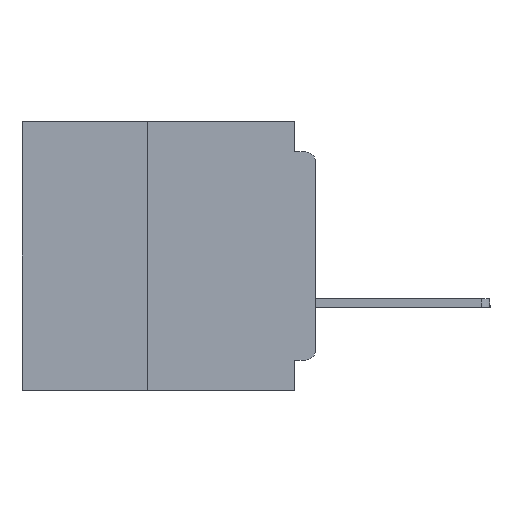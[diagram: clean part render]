
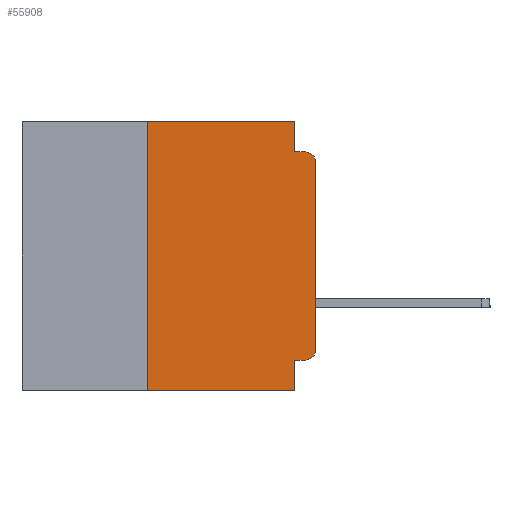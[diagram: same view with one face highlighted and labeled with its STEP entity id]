
A CAD part, left-side view. The second image highlights one B-rep face of the part: STEP entity #55908.
In plain terms, the highlighted planar face has unit normal (-1, 0, 0).
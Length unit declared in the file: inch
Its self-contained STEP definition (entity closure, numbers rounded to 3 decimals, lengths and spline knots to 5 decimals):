
#20 = VERTEX_POINT ( 'NONE', #24522 ) ;
#224 = CARTESIAN_POINT ( 'NONE',  ( 0., 0.015, -0.06 ) ) ;
#726 = LINE ( 'NONE', #30861, #12191 ) ;
#818 = CARTESIAN_POINT ( 'NONE',  ( 0., 0.437, 0. ) ) ;
#1888 = DIRECTION ( 'NONE',  ( 0., -1., 0. ) ) ;
#3076 = ORIENTED_EDGE ( 'NONE', *, *, #14187, .F. ) ;
#3873 = VERTEX_POINT ( 'NONE', #3890 ) ;
#3890 = CARTESIAN_POINT ( 'NONE',  ( 0., 0., -0.06 ) ) ;
#4310 = DIRECTION ( 'NONE',  ( -1., 0., 0. ) ) ;
#5172 = DIRECTION ( 'NONE',  ( 0., 0., -1. ) ) ;
#5753 = DIRECTION ( 'NONE',  ( 0., 0., -1. ) ) ;
#6832 = ORIENTED_EDGE ( 'NONE', *, *, #9218, .F. ) ;
#8948 = VERTEX_POINT ( 'NONE', #24760 ) ;
#9218 = EDGE_CURVE ( 'NONE', #56957, #15188, #60233, .T. ) ;
#9651 = VECTOR ( 'NONE', #26650, 39.37008 ) ;
#9914 = VERTEX_POINT ( 'NONE', #55533 ) ;
#10625 = ORIENTED_EDGE ( 'NONE', *, *, #50321, .F. ) ;
#11396 = ORIENTED_EDGE ( 'NONE', *, *, #52573, .F. ) ;
#12191 = VECTOR ( 'NONE', #16539, 39.37008 ) ;
#12241 = EDGE_CURVE ( 'NONE', #8948, #20674, #726, .T. ) ;
#12312 = CARTESIAN_POINT ( 'NONE',  ( 0., 0., -0.355 ) ) ;
#12936 = EDGE_LOOP ( 'NONE', ( #21149, #47153, #47600, #10625, #11396, #6832, #40379, #48515, #3076, #17005 ) ) ;
#14187 = EDGE_CURVE ( 'NONE', #20, #8948, #46287, .T. ) ;
#14747 = CARTESIAN_POINT ( 'NONE',  ( 0., 0.031, -0.4 ) ) ;
#15188 = VERTEX_POINT ( 'NONE', #15337 ) ;
#15337 = CARTESIAN_POINT ( 'NONE',  ( 0., 0.25, 0. ) ) ;
#16345 = CARTESIAN_POINT ( 'NONE',  ( 0., 0., -0.045 ) ) ;
#16539 = DIRECTION ( 'NONE',  ( 0., 0., -1. ) ) ;
#17005 = ORIENTED_EDGE ( 'NONE', *, *, #46021, .T. ) ;
#20462 = LINE ( 'NONE', #60991, #55417 ) ;
#20674 = VERTEX_POINT ( 'NONE', #14747 ) ;
#21149 = ORIENTED_EDGE ( 'NONE', *, *, #46573, .T. ) ;
#21514 = EDGE_CURVE ( 'NONE', #9914, #60119, #39062, .T. ) ;
#22411 = VECTOR ( 'NONE', #31202, 39.37008 ) ;
#24050 = CARTESIAN_POINT ( 'NONE',  ( 0., 0.031, 0. ) ) ;
#24522 = CARTESIAN_POINT ( 'NONE',  ( 0., 0.015, -0.355 ) ) ;
#24693 = AXIS2_PLACEMENT_3D ( 'NONE', #33201, #4310, #37907 ) ;
#24760 = CARTESIAN_POINT ( 'NONE',  ( 0., 0.031, -0.355 ) ) ;
#26650 = DIRECTION ( 'NONE',  ( 0., 1., 0. ) ) ;
#28067 = CIRCLE ( 'NONE', #24693, 0.015 ) ;
#30284 = CIRCLE ( 'NONE', #51730, 0.015 ) ;
#30861 = CARTESIAN_POINT ( 'NONE',  ( 0., 0.031, -0.4 ) ) ;
#31202 = DIRECTION ( 'NONE',  ( 0., 0., 1. ) ) ;
#32042 = VERTEX_POINT ( 'NONE', #36938 ) ;
#32251 = LINE ( 'NONE', #24050, #55947 ) ;
#32519 = FACE_OUTER_BOUND ( 'NONE', #12936, .T. ) ;
#33201 = CARTESIAN_POINT ( 'NONE',  ( 0., 0.015, -0.34 ) ) ;
#33380 = DIRECTION ( 'NONE',  ( 0., -1., 0. ) ) ;
#33451 = VERTEX_POINT ( 'NONE', #48397 ) ;
#34052 = DIRECTION ( 'NONE',  ( -1., 0., 0. ) ) ;
#34593 = DIRECTION ( 'NONE',  ( 1., 0., 0. ) ) ;
#36938 = CARTESIAN_POINT ( 'NONE',  ( 0., 0., -0.34 ) ) ;
#37600 = VECTOR ( 'NONE', #1888, 39.37008 ) ;
#37907 = DIRECTION ( 'NONE',  ( 0., 0., -1. ) ) ;
#38550 = LINE ( 'NONE', #61639, #52707 ) ;
#39062 = LINE ( 'NONE', #16345, #37600 ) ;
#40379 = ORIENTED_EDGE ( 'NONE', *, *, #50303, .T. ) ;
#42589 = CARTESIAN_POINT ( 'NONE',  ( 0., 0.25, -0.4 ) ) ;
#43117 = DIRECTION ( 'NONE',  ( 0., 0., -1. ) ) ;
#46021 = EDGE_CURVE ( 'NONE', #20, #32042, #28067, .T. ) ;
#46287 = LINE ( 'NONE', #12312, #9651 ) ;
#46304 = LINE ( 'NONE', #47697, #57376 ) ;
#46573 = EDGE_CURVE ( 'NONE', #32042, #3873, #20462, .T. ) ;
#47153 = ORIENTED_EDGE ( 'NONE', *, *, #59914, .T. ) ;
#47600 = ORIENTED_EDGE ( 'NONE', *, *, #21514, .F. ) ;
#47697 = CARTESIAN_POINT ( 'NONE',  ( 0., 0.437, -0.4 ) ) ;
#48397 = CARTESIAN_POINT ( 'NONE',  ( 0., 0.031, 0. ) ) ;
#48515 = ORIENTED_EDGE ( 'NONE', *, *, #12241, .F. ) ;
#50303 = EDGE_CURVE ( 'NONE', #56957, #20674, #46304, .T. ) ;
#50321 = EDGE_CURVE ( 'NONE', #33451, #9914, #32251, .T. ) ;
#51730 = AXIS2_PLACEMENT_3D ( 'NONE', #224, #34052, #5172 ) ;
#52505 = DIRECTION ( 'NONE',  ( 0., -1., 0. ) ) ;
#52573 = EDGE_CURVE ( 'NONE', #15188, #33451, #38550, .T. ) ;
#52707 = VECTOR ( 'NONE', #33380, 39.37008 ) ;
#55305 = AXIS2_PLACEMENT_3D ( 'NONE', #818, #34593, #5753 ) ;
#55417 = VECTOR ( 'NONE', #56299, 39.37008 ) ;
#55533 = CARTESIAN_POINT ( 'NONE',  ( 0., 0.031, -0.045 ) ) ;
#55908 = ADVANCED_FACE ( 'NONE', ( #32519 ), #58139, .F. ) ;
#55947 = VECTOR ( 'NONE', #43117, 39.37008 ) ;
#56299 = DIRECTION ( 'NONE',  ( 0., 0., 1. ) ) ;
#56957 = VERTEX_POINT ( 'NONE', #42589 ) ;
#57376 = VECTOR ( 'NONE', #52505, 39.37008 ) ;
#58139 = PLANE ( 'NONE',  #55305 ) ;
#59400 = CARTESIAN_POINT ( 'NONE',  ( 0., 0.015, -0.045 ) ) ;
#59491 = CARTESIAN_POINT ( 'NONE',  ( 0., 0.25, -0.4 ) ) ;
#59914 = EDGE_CURVE ( 'NONE', #3873, #60119, #30284, .T. ) ;
#60119 = VERTEX_POINT ( 'NONE', #59400 ) ;
#60233 = LINE ( 'NONE', #59491, #22411 ) ;
#60991 = CARTESIAN_POINT ( 'NONE',  ( 0., 0., 0. ) ) ;
#61639 = CARTESIAN_POINT ( 'NONE',  ( 0., 0.437, 0. ) ) ;
